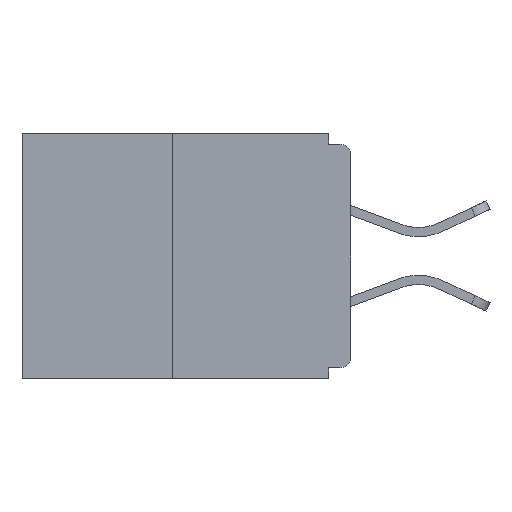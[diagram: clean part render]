
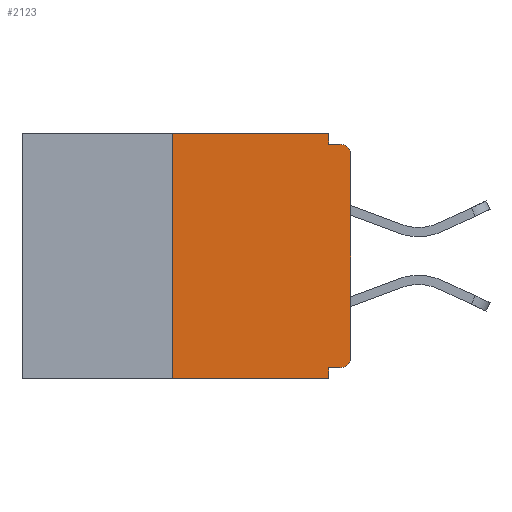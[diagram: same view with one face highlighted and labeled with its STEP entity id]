
A CAD part, left-side view. The second image highlights one B-rep face of the part: STEP entity #2123.
In plain terms, the highlighted planar face has unit normal (-1, 0, 0).
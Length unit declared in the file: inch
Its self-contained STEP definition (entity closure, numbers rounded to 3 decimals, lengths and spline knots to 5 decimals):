
#64 = EDGE_CURVE ( 'NONE', #4904, #5939, #8788, .T. ) ;
#293 = DIRECTION ( 'NONE',  ( 0., 0., 1. ) ) ;
#338 = CARTESIAN_POINT ( 'NONE',  ( 0., 0., -0.015 ) ) ;
#466 = CARTESIAN_POINT ( 'NONE',  ( 0., 0.031, 0. ) ) ;
#497 = ORIENTED_EDGE ( 'NONE', *, *, #5548, .F. ) ;
#706 = CARTESIAN_POINT ( 'NONE',  ( 0., 0.015, -0.313 ) ) ;
#751 = EDGE_CURVE ( 'NONE', #11116, #3069, #13006, .T. ) ;
#1058 = AXIS2_PLACEMENT_3D ( 'NONE', #706, #7375, #1949 ) ;
#1083 = AXIS2_PLACEMENT_3D ( 'NONE', #6456, #3333, #12055 ) ;
#1241 = VECTOR ( 'NONE', #12420, 39.37008 ) ;
#1305 = CARTESIAN_POINT ( 'NONE',  ( 0., 0., 0. ) ) ;
#1575 = ORIENTED_EDGE ( 'NONE', *, *, #751, .T. ) ;
#1890 = ORIENTED_EDGE ( 'NONE', *, *, #9999, .F. ) ;
#1928 = LINE ( 'NONE', #4549, #13290 ) ;
#1949 = DIRECTION ( 'NONE',  ( 0., 0., -1. ) ) ;
#2015 = VERTEX_POINT ( 'NONE', #11860 ) ;
#2123 = ADVANCED_FACE ( 'NONE', ( #8376 ), #13032, .F. ) ;
#2565 = DIRECTION ( 'NONE',  ( 0., 0., 1. ) ) ;
#2747 = VECTOR ( 'NONE', #293, 39.37008 ) ;
#2882 = VECTOR ( 'NONE', #3153, 39.37008 ) ;
#3069 = VERTEX_POINT ( 'NONE', #12121 ) ;
#3070 = ORIENTED_EDGE ( 'NONE', *, *, #4823, .F. ) ;
#3153 = DIRECTION ( 'NONE',  ( 0., 1., 0. ) ) ;
#3214 = EDGE_CURVE ( 'NONE', #2015, #3461, #1928, .T. ) ;
#3333 = DIRECTION ( 'NONE',  ( 1., 0., 0. ) ) ;
#3415 = LINE ( 'NONE', #13516, #10803 ) ;
#3461 = VERTEX_POINT ( 'NONE', #3974 ) ;
#3653 = AXIS2_PLACEMENT_3D ( 'NONE', #7262, #8436, #8525 ) ;
#3974 = CARTESIAN_POINT ( 'NONE',  ( 0., 0.031, -0.343 ) ) ;
#4003 = ORIENTED_EDGE ( 'NONE', *, *, #7125, .F. ) ;
#4027 = VECTOR ( 'NONE', #7837, 39.37008 ) ;
#4310 = CARTESIAN_POINT ( 'NONE',  ( 0., 0.031, -0.328 ) ) ;
#4453 = EDGE_LOOP ( 'NONE', ( #11300, #497, #6462, #3070, #12924, #12932, #13602, #1575, #4003, #1890 ) ) ;
#4549 = CARTESIAN_POINT ( 'NONE',  ( 0., 0.46, -0.343 ) ) ;
#4598 = DIRECTION ( 'NONE',  ( 0., -1., 0. ) ) ;
#4823 = EDGE_CURVE ( 'NONE', #14106, #3461, #11670, .T. ) ;
#4904 = VERTEX_POINT ( 'NONE', #8872 ) ;
#5008 = EDGE_CURVE ( 'NONE', #5939, #11116, #5999, .T. ) ;
#5097 = CARTESIAN_POINT ( 'NONE',  ( 0., 0.031, -0.343 ) ) ;
#5165 = VERTEX_POINT ( 'NONE', #13498 ) ;
#5427 = LINE ( 'NONE', #338, #13861 ) ;
#5548 = EDGE_CURVE ( 'NONE', #2015, #5165, #3415, .T. ) ;
#5934 = CARTESIAN_POINT ( 'NONE',  ( 0., 0.031, -0.015 ) ) ;
#5939 = VERTEX_POINT ( 'NONE', #6469 ) ;
#5999 = LINE ( 'NONE', #1305, #2747 ) ;
#6456 = CARTESIAN_POINT ( 'NONE',  ( 0., 0.46, 0. ) ) ;
#6462 = ORIENTED_EDGE ( 'NONE', *, *, #3214, .T. ) ;
#6469 = CARTESIAN_POINT ( 'NONE',  ( 0., 0., -0.313 ) ) ;
#6732 = EDGE_CURVE ( 'NONE', #4904, #14106, #13874, .T. ) ;
#7125 = EDGE_CURVE ( 'NONE', #12613, #3069, #5427, .T. ) ;
#7229 = VERTEX_POINT ( 'NONE', #466 ) ;
#7262 = CARTESIAN_POINT ( 'NONE',  ( 0., 0.015, -0.03 ) ) ;
#7375 = DIRECTION ( 'NONE',  ( -1., 0., 0. ) ) ;
#7837 = DIRECTION ( 'NONE',  ( 0., -1., 0. ) ) ;
#8376 = FACE_OUTER_BOUND ( 'NONE', #4453, .T. ) ;
#8436 = DIRECTION ( 'NONE',  ( -1., 0., 0. ) ) ;
#8525 = DIRECTION ( 'NONE',  ( 0., 0., -1. ) ) ;
#8624 = EDGE_CURVE ( 'NONE', #5165, #7229, #10045, .T. ) ;
#8788 = CIRCLE ( 'NONE', #1058, 0.015 ) ;
#8872 = CARTESIAN_POINT ( 'NONE',  ( 0., 0.015, -0.328 ) ) ;
#9307 = CARTESIAN_POINT ( 'NONE',  ( 0., 0.031, 0. ) ) ;
#9524 = DIRECTION ( 'NONE',  ( 0., 0., -1. ) ) ;
#9635 = CARTESIAN_POINT ( 'NONE',  ( 0., 0., -0.03 ) ) ;
#9999 = EDGE_CURVE ( 'NONE', #7229, #12613, #10529, .T. ) ;
#10045 = LINE ( 'NONE', #13401, #4027 ) ;
#10482 = VECTOR ( 'NONE', #9524, 39.37008 ) ;
#10529 = LINE ( 'NONE', #9307, #1241 ) ;
#10803 = VECTOR ( 'NONE', #2565, 39.37008 ) ;
#11116 = VERTEX_POINT ( 'NONE', #9635 ) ;
#11300 = ORIENTED_EDGE ( 'NONE', *, *, #8624, .F. ) ;
#11670 = LINE ( 'NONE', #5097, #10482 ) ;
#11860 = CARTESIAN_POINT ( 'NONE',  ( 0., 0.25, -0.343 ) ) ;
#12055 = DIRECTION ( 'NONE',  ( 0., 0., -1. ) ) ;
#12121 = CARTESIAN_POINT ( 'NONE',  ( 0., 0.015, -0.015 ) ) ;
#12420 = DIRECTION ( 'NONE',  ( 0., 0., -1. ) ) ;
#12544 = DIRECTION ( 'NONE',  ( 0., -1., 0. ) ) ;
#12613 = VERTEX_POINT ( 'NONE', #5934 ) ;
#12924 = ORIENTED_EDGE ( 'NONE', *, *, #6732, .F. ) ;
#12932 = ORIENTED_EDGE ( 'NONE', *, *, #64, .T. ) ;
#13006 = CIRCLE ( 'NONE', #3653, 0.015 ) ;
#13032 = PLANE ( 'NONE',  #1083 ) ;
#13290 = VECTOR ( 'NONE', #4598, 39.37008 ) ;
#13401 = CARTESIAN_POINT ( 'NONE',  ( 0., 0.46, 0. ) ) ;
#13498 = CARTESIAN_POINT ( 'NONE',  ( 0., 0.25, 0. ) ) ;
#13516 = CARTESIAN_POINT ( 'NONE',  ( 0., 0.25, 0. ) ) ;
#13602 = ORIENTED_EDGE ( 'NONE', *, *, #5008, .T. ) ;
#13861 = VECTOR ( 'NONE', #12544, 39.37008 ) ;
#13874 = LINE ( 'NONE', #14100, #2882 ) ;
#14100 = CARTESIAN_POINT ( 'NONE',  ( 0., 0., -0.328 ) ) ;
#14106 = VERTEX_POINT ( 'NONE', #4310 ) ;
